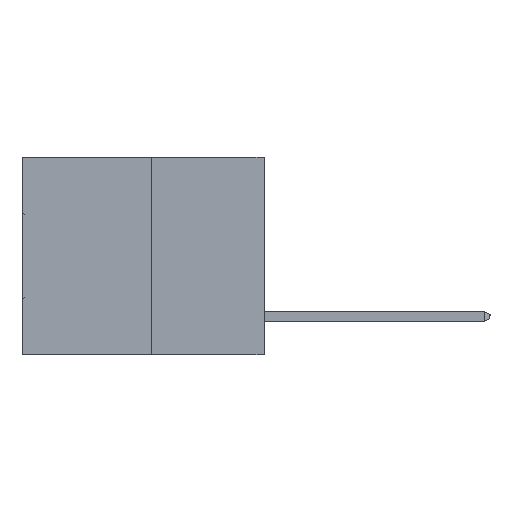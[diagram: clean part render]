
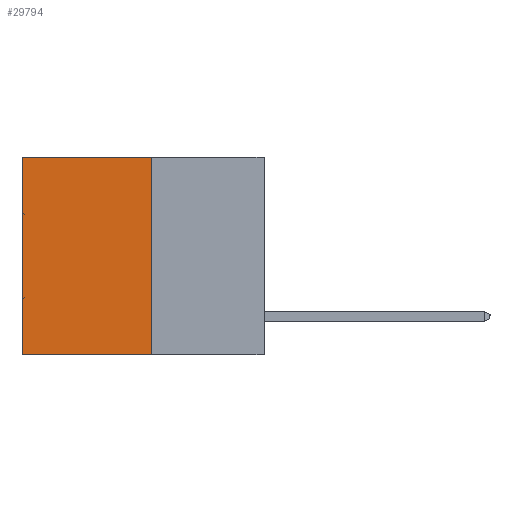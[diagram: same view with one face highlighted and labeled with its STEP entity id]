
A CAD part, left-side view. The second image highlights one B-rep face of the part: STEP entity #29794.
In plain terms, the highlighted planar face has unit normal (-1, 0, 0).
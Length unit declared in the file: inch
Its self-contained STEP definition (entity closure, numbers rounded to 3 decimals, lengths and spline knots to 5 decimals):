
#596 = CARTESIAN_POINT ( 'NONE',  ( 0.3165, 0.28, -0.49 ) ) ;
#1127 = DIRECTION ( 'NONE',  ( 0., 0., -1. ) ) ;
#1915 = CARTESIAN_POINT ( 'NONE',  ( 0.3165, 0.6, -0.49 ) ) ;
#2616 = VERTEX_POINT ( 'NONE', #28382 ) ;
#3203 = EDGE_CURVE ( 'NONE', #33379, #2616, #17665, .T. ) ;
#4232 = DIRECTION ( 'NONE',  ( 0., 0., -1. ) ) ;
#4331 = ORIENTED_EDGE ( 'NONE', *, *, #31657, .T. ) ;
#4597 = EDGE_CURVE ( 'NONE', #22948, #33379, #11663, .T. ) ;
#5383 = DIRECTION ( 'NONE',  ( 0., 1., 0. ) ) ;
#6298 = CARTESIAN_POINT ( 'NONE',  ( 0.3165, 0.28, -0.49 ) ) ;
#8410 = VECTOR ( 'NONE', #11122, 39.37008 ) ;
#9062 = VECTOR ( 'NONE', #15861, 39.37008 ) ;
#9250 = PLANE ( 'NONE',  #23161 ) ;
#11109 = LINE ( 'NONE', #34551, #12808 ) ;
#11122 = DIRECTION ( 'NONE',  ( 0., 1., 0. ) ) ;
#11299 = ORIENTED_EDGE ( 'NONE', *, *, #4597, .F. ) ;
#11663 = LINE ( 'NONE', #25774, #25572 ) ;
#11941 = ORIENTED_EDGE ( 'NONE', *, *, #3203, .F. ) ;
#12808 = VECTOR ( 'NONE', #5383, 39.37008 ) ;
#15861 = DIRECTION ( 'NONE',  ( 0., 0., -1. ) ) ;
#17665 = LINE ( 'NONE', #32658, #8410 ) ;
#21264 = EDGE_LOOP ( 'NONE', ( #4331, #11941, #11299, #30843 ) ) ;
#22557 = DIRECTION ( 'NONE',  ( 1., 0., 0. ) ) ;
#22948 = VERTEX_POINT ( 'NONE', #33274 ) ;
#23161 = AXIS2_PLACEMENT_3D ( 'NONE', #6298, #22557, #1127 ) ;
#25572 = VECTOR ( 'NONE', #4232, 39.37008 ) ;
#25774 = CARTESIAN_POINT ( 'NONE',  ( 0.3165, 0.28, -0.49 ) ) ;
#26710 = CARTESIAN_POINT ( 'NONE',  ( 0.3165, 0.6, 0. ) ) ;
#28154 = VERTEX_POINT ( 'NONE', #26710 ) ;
#28382 = CARTESIAN_POINT ( 'NONE',  ( 0.3165, 0.6, -0.49 ) ) ;
#28451 = LINE ( 'NONE', #1915, #9062 ) ;
#29203 = EDGE_CURVE ( 'NONE', #22948, #28154, #11109, .T. ) ;
#29794 = ADVANCED_FACE ( 'NONE', ( #32988 ), #9250, .F. ) ;
#30843 = ORIENTED_EDGE ( 'NONE', *, *, #29203, .T. ) ;
#31657 = EDGE_CURVE ( 'NONE', #28154, #2616, #28451, .T. ) ;
#32658 = CARTESIAN_POINT ( 'NONE',  ( 0.3165, 0.28, -0.49 ) ) ;
#32988 = FACE_OUTER_BOUND ( 'NONE', #21264, .T. ) ;
#33274 = CARTESIAN_POINT ( 'NONE',  ( 0.3165, 0.28, 0. ) ) ;
#33379 = VERTEX_POINT ( 'NONE', #596 ) ;
#34551 = CARTESIAN_POINT ( 'NONE',  ( 0.3165, 0.28, 0. ) ) ;
